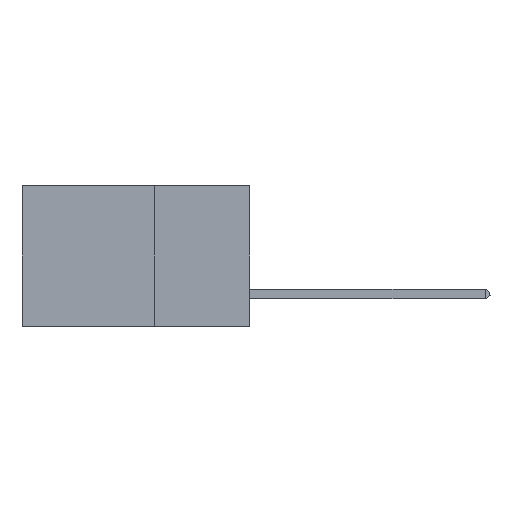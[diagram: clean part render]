
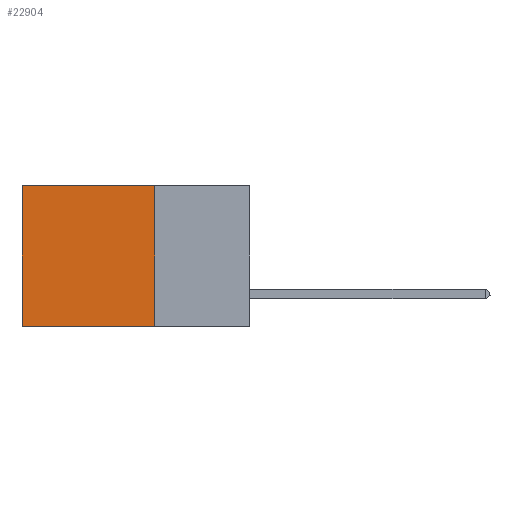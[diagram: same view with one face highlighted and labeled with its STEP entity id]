
A CAD part, left-side view. The second image highlights one B-rep face of the part: STEP entity #22904.
In plain terms, the highlighted planar face has unit normal (-1, 0, 0).
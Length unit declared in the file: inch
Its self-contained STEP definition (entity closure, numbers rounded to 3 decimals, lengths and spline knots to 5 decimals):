
#77 = LINE ( 'NONE', #22655, #2282 ) ;
#483 = CARTESIAN_POINT ( 'NONE',  ( 0.2875, 0.25, 0. ) ) ;
#999 = CARTESIAN_POINT ( 'NONE',  ( 0.2875, 0.25, -0.37 ) ) ;
#1197 = AXIS2_PLACEMENT_3D ( 'NONE', #1844, #29820, #8869 ) ;
#1844 = CARTESIAN_POINT ( 'NONE',  ( 0.2875, 0.25, 0. ) ) ;
#2282 = VECTOR ( 'NONE', #8342, 39.37008 ) ;
#3149 = DIRECTION ( 'NONE',  ( 0., 1., 0. ) ) ;
#7810 = LINE ( 'NONE', #17181, #39450 ) ;
#8342 = DIRECTION ( 'NONE',  ( 0., 0., -1. ) ) ;
#8792 = EDGE_CURVE ( 'NONE', #20793, #20396, #7810, .T. ) ;
#8869 = DIRECTION ( 'NONE',  ( 0., 0., -1. ) ) ;
#10455 = VERTEX_POINT ( 'NONE', #13094 ) ;
#12229 = LINE ( 'NONE', #34282, #18213 ) ;
#13094 = CARTESIAN_POINT ( 'NONE',  ( 0.2875, 0.25, -0.37 ) ) ;
#14570 = FACE_OUTER_BOUND ( 'NONE', #30118, .T. ) ;
#17181 = CARTESIAN_POINT ( 'NONE',  ( 0.2875, 0.25, 0. ) ) ;
#17211 = ORIENTED_EDGE ( 'NONE', *, *, #8792, .T. ) ;
#17316 = DIRECTION ( 'NONE',  ( 0., 0., -1. ) ) ;
#18213 = VECTOR ( 'NONE', #17316, 39.37008 ) ;
#20396 = VERTEX_POINT ( 'NONE', #33801 ) ;
#20793 = VERTEX_POINT ( 'NONE', #483 ) ;
#22655 = CARTESIAN_POINT ( 'NONE',  ( 0.2875, 0.6, 0. ) ) ;
#22904 = ADVANCED_FACE ( 'NONE', ( #14570 ), #33174, .F. ) ;
#26376 = EDGE_CURVE ( 'NONE', #20396, #43267, #77, .T. ) ;
#28526 = ORIENTED_EDGE ( 'NONE', *, *, #30937, .F. ) ;
#29719 = CARTESIAN_POINT ( 'NONE',  ( 0.2875, 0.6, -0.37 ) ) ;
#29820 = DIRECTION ( 'NONE',  ( 1., 0., 0. ) ) ;
#30118 = EDGE_LOOP ( 'NONE', ( #37938, #35707, #28526, #17211 ) ) ;
#30937 = EDGE_CURVE ( 'NONE', #20793, #10455, #12229, .T. ) ;
#32309 = DIRECTION ( 'NONE',  ( 0., 1., 0. ) ) ;
#32644 = LINE ( 'NONE', #999, #33733 ) ;
#33174 = PLANE ( 'NONE',  #1197 ) ;
#33733 = VECTOR ( 'NONE', #32309, 39.37008 ) ;
#33801 = CARTESIAN_POINT ( 'NONE',  ( 0.2875, 0.6, 0. ) ) ;
#34282 = CARTESIAN_POINT ( 'NONE',  ( 0.2875, 0.25, 0. ) ) ;
#35707 = ORIENTED_EDGE ( 'NONE', *, *, #40004, .F. ) ;
#37938 = ORIENTED_EDGE ( 'NONE', *, *, #26376, .T. ) ;
#39450 = VECTOR ( 'NONE', #3149, 39.37008 ) ;
#40004 = EDGE_CURVE ( 'NONE', #10455, #43267, #32644, .T. ) ;
#43267 = VERTEX_POINT ( 'NONE', #29719 ) ;
